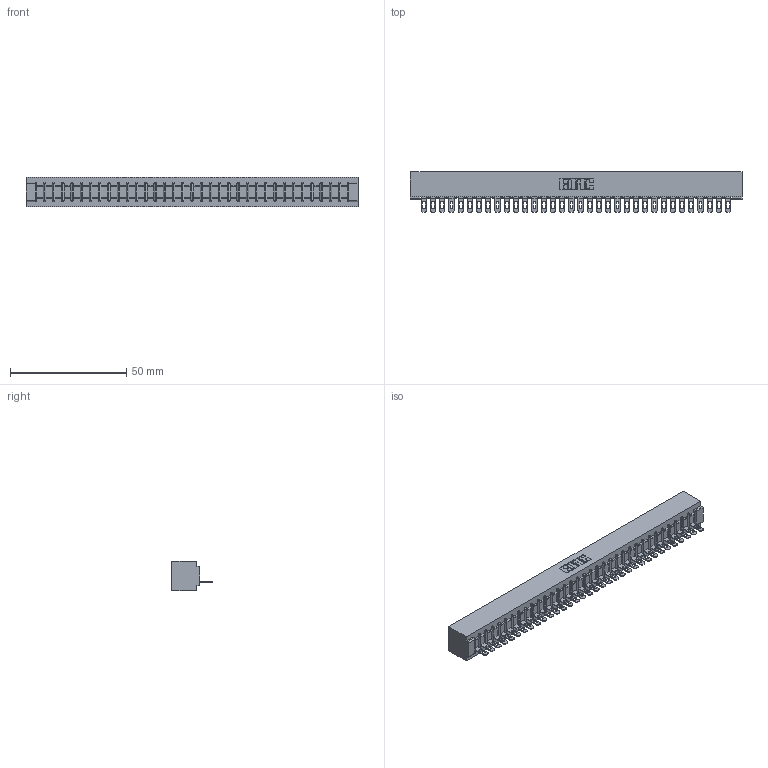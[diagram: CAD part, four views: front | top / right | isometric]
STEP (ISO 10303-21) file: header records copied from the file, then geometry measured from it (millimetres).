
FILE_DESCRIPTION (( 'STEP AP203' ), '1' );
FILE_NAME ('307-034-401-101.STEP', '2020-09-28T21:05:41', ( '' ), ( '' ), 'SwSTEP 2.0', 'SolidWorks 2020', '' );
FILE_SCHEMA (( 'CONFIG_CONTROL_DESIGN' ));
Length unit declared in the file: inch
Products named in the file (3): 307-034-401-101; 307-290-002_501; 307 Part_No Mounting Lugs
Assembly tree (35 placements, depth 2):
  307-034-401-101
    307 Part_No Mounting Lugs
    307-290-002_501  x34
Bounding box: 142.6 x 17.42 x 12.7 mm (x, y, z)
Volume: 15787.3 mm3; surface area: 20254.4 mm2
Topology: 35 solids, 35 shells, 2729 faces, 8391 edges, 5498 vertices
Faces by surface type: plane 1562, cylinder 1097, sphere 70
Entity records: 30650 total; most frequent: CARTESIAN_POINT 5168, ORIENTED_EDGE 5158, DIRECTION 5027, EDGE_CURVE 2579, VECTOR 1969, LINE 1969, VERTEX_POINT 1670, AXIS2_PLACEMENT_3D 1529
